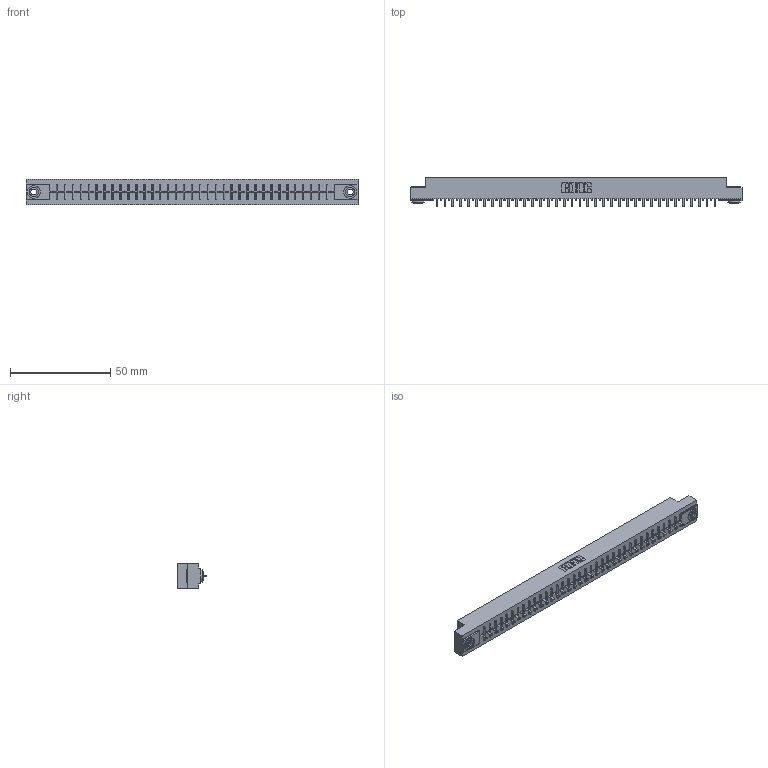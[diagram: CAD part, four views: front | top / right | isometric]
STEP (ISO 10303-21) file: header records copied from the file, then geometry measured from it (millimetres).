
FILE_DESCRIPTION (( 'STEP AP203' ), '1' );
FILE_NAME ('316-036-521-103.STEP', '2018-07-31T04:32:20', ( '' ), ( '' ), 'SwSTEP 2.0', 'SolidWorks 2016', '' );
FILE_SCHEMA (( 'CONFIG_CONTROL_DESIGN' ));
Length unit declared in the file: inch
Products named in the file (4): 316-036-521-103; 306 Part_.156 Dia; 306-290-001_121; 345-250-002_345-250-002-102
Assembly tree (39 placements, depth 2):
  316-036-521-103
    306 Part_.156 Dia
    306-290-001_121  x36
    345-250-002_345-250-002-102  x2
Bounding box: 165.66 x 14.88 x 12.7 mm (x, y, z)
Volume: 18226.9 mm3; surface area: 18624.2 mm2
Topology: 39 solids, 39 shells, 2688 faces, 7520 edges, 4816 vertices
Faces by surface type: plane 1784, cylinder 752, sphere 144, cone 8
Entity records: 35370 total; most frequent: CARTESIAN_POINT 5916, ORIENTED_EDGE 5856, DIRECTION 5848, EDGE_CURVE 2928, VECTOR 2280, LINE 2280, VERTEX_POINT 1852, AXIS2_PLACEMENT_3D 1784
